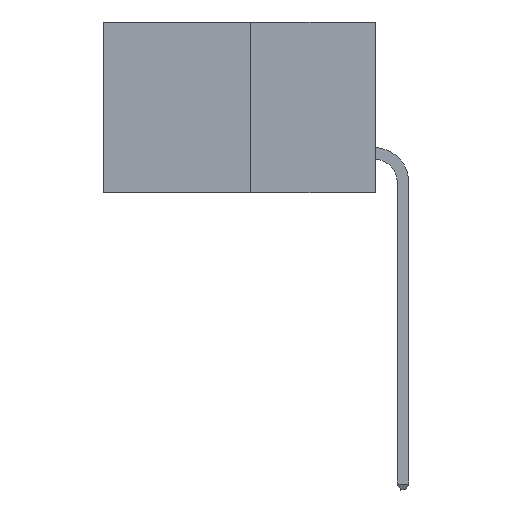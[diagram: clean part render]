
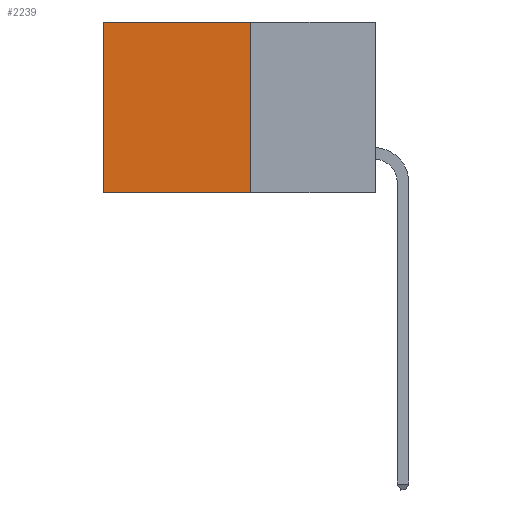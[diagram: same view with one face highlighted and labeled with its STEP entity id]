
A CAD part, left-side view. The second image highlights one B-rep face of the part: STEP entity #2239.
In plain terms, the highlighted planar face has unit normal (-1, 0, 0).
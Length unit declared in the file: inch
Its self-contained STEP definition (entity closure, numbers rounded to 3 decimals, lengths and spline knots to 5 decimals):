
#88 = ORIENTED_EDGE ( 'NONE', *, *, #9960, .T. ) ;
#341 = ORIENTED_EDGE ( 'NONE', *, *, #2309, .F. ) ;
#498 = VECTOR ( 'NONE', #4618, 39.37008 ) ;
#1072 = CARTESIAN_POINT ( 'NONE',  ( 0.277, 0.27, -0.37 ) ) ;
#1176 = DIRECTION ( 'NONE',  ( 0., 0., -1. ) ) ;
#1331 = VERTEX_POINT ( 'NONE', #1072 ) ;
#1831 = VERTEX_POINT ( 'NONE', #3044 ) ;
#2239 = ADVANCED_FACE ( 'NONE', ( #10224 ), #5987, .F. ) ;
#2241 = EDGE_CURVE ( 'NONE', #1331, #3796, #9730, .T. ) ;
#2282 = CARTESIAN_POINT ( 'NONE',  ( 0.277, 0.27, 0. ) ) ;
#2309 = EDGE_CURVE ( 'NONE', #2778, #1331, #2933, .T. ) ;
#2535 = ORIENTED_EDGE ( 'NONE', *, *, #8699, .T. ) ;
#2655 = DIRECTION ( 'NONE',  ( 1., 0., 0. ) ) ;
#2769 = DIRECTION ( 'NONE',  ( 0., 1., 0. ) ) ;
#2778 = VERTEX_POINT ( 'NONE', #9106 ) ;
#2933 = LINE ( 'NONE', #5234, #7103 ) ;
#3044 = CARTESIAN_POINT ( 'NONE',  ( 0.277, 0.59, 0. ) ) ;
#3796 = VERTEX_POINT ( 'NONE', #7833 ) ;
#4505 = VECTOR ( 'NONE', #7278, 39.37008 ) ;
#4618 = DIRECTION ( 'NONE',  ( 0., 0., -1. ) ) ;
#5026 = LINE ( 'NONE', #2282, #4505 ) ;
#5059 = LINE ( 'NONE', #9508, #498 ) ;
#5234 = CARTESIAN_POINT ( 'NONE',  ( 0.277, 0.27, -0.37 ) ) ;
#5678 = VECTOR ( 'NONE', #2769, 39.37008 ) ;
#5707 = AXIS2_PLACEMENT_3D ( 'NONE', #7487, #2655, #1176 ) ;
#5987 = PLANE ( 'NONE',  #5707 ) ;
#7103 = VECTOR ( 'NONE', #9202, 39.37008 ) ;
#7278 = DIRECTION ( 'NONE',  ( 0., 1., 0. ) ) ;
#7487 = CARTESIAN_POINT ( 'NONE',  ( 0.277, 0.27, -0.37 ) ) ;
#7767 = CARTESIAN_POINT ( 'NONE',  ( 0.277, 0.27, -0.37 ) ) ;
#7833 = CARTESIAN_POINT ( 'NONE',  ( 0.277, 0.59, -0.37 ) ) ;
#8699 = EDGE_CURVE ( 'NONE', #1831, #3796, #5059, .T. ) ;
#9106 = CARTESIAN_POINT ( 'NONE',  ( 0.277, 0.27, 0. ) ) ;
#9202 = DIRECTION ( 'NONE',  ( 0., 0., -1. ) ) ;
#9508 = CARTESIAN_POINT ( 'NONE',  ( 0.277, 0.59, -0.37 ) ) ;
#9730 = LINE ( 'NONE', #7767, #5678 ) ;
#9916 = ORIENTED_EDGE ( 'NONE', *, *, #2241, .F. ) ;
#9960 = EDGE_CURVE ( 'NONE', #2778, #1831, #5026, .T. ) ;
#10224 = FACE_OUTER_BOUND ( 'NONE', #10249, .T. ) ;
#10249 = EDGE_LOOP ( 'NONE', ( #2535, #9916, #341, #88 ) ) ;
